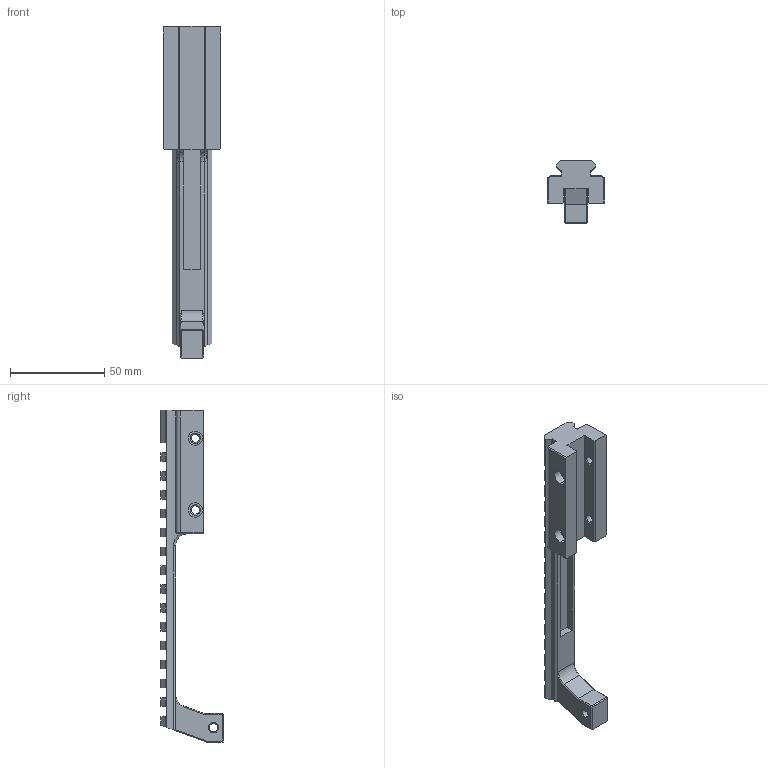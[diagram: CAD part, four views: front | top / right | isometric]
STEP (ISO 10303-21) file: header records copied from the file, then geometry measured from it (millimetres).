
FILE_DESCRIPTION (( 'STEP AP214' ), '1' );
FILE_NAME ('Optic Rail.STEP', '2022-02-04T02:40:26', ( '' ), ( '' ), 'SwSTEP 2.0', 'SolidWorks 2020', '' );
FILE_SCHEMA (( 'AUTOMOTIVE_DESIGN' ));
Length unit declared in the file: inch
Products named in the file (1): Optic Rail
Bounding box: 30.42 x 32.95 x 176.28 mm (x, y, z)
Volume: 43399.1 mm3; surface area: 18351.5 mm2
Topology: 1 solids, 1 shells, 204 faces, 558 edges, 360 vertices
Faces by surface type: plane 165, cone 20, cylinder 19
Entity records: 6404 total; most frequent: CARTESIAN_POINT 1143, ORIENTED_EDGE 1116, DIRECTION 1022, EDGE_CURVE 558, VECTOR 496, LINE 496, VERTEX_POINT 360, AXIS2_PLACEMENT_3D 263
